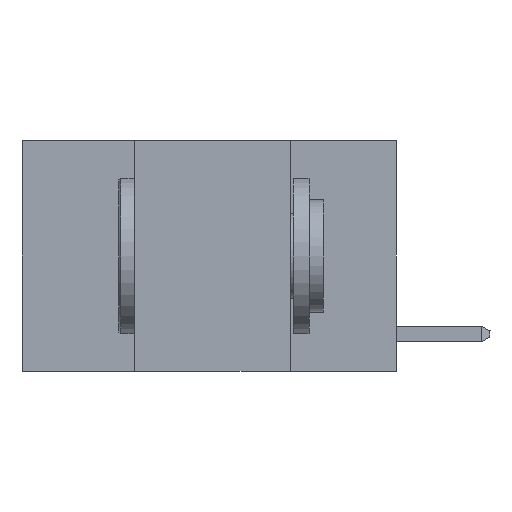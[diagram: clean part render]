
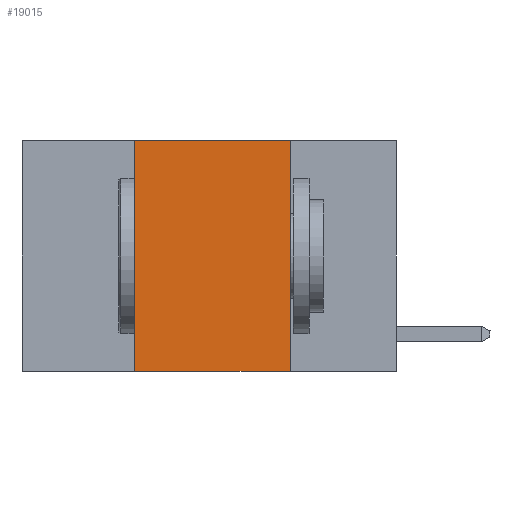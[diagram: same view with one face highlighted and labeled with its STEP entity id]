
A CAD part, left-side view. The second image highlights one B-rep face of the part: STEP entity #19015.
In plain terms, the highlighted planar face has unit normal (-1, 0, 0).
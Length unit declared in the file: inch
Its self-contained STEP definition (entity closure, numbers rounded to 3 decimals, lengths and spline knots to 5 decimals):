
#1321 = CARTESIAN_POINT ( 'NONE',  ( 0., 0.17, -0.37 ) ) ;
#1648 = EDGE_CURVE ( 'NONE', #19116, #20212, #13158, .T. ) ;
#2033 = CARTESIAN_POINT ( 'NONE',  ( 0., 0.42, -0.37 ) ) ;
#2438 = CARTESIAN_POINT ( 'NONE',  ( 0., 0.17, 0. ) ) ;
#2648 = VERTEX_POINT ( 'NONE', #1321 ) ;
#3921 = ORIENTED_EDGE ( 'NONE', *, *, #10021, .F. ) ;
#4187 = VERTEX_POINT ( 'NONE', #17325 ) ;
#4272 = ORIENTED_EDGE ( 'NONE', *, *, #1648, .F. ) ;
#4776 = VECTOR ( 'NONE', #13608, 39.37008 ) ;
#5179 = CARTESIAN_POINT ( 'NONE',  ( 0., 0.42, 0. ) ) ;
#5479 = DIRECTION ( 'NONE',  ( 0., 0., -1. ) ) ;
#6672 = PLANE ( 'NONE',  #11366 ) ;
#7063 = CARTESIAN_POINT ( 'NONE',  ( 0., 0.6, -0.37 ) ) ;
#7720 = ORIENTED_EDGE ( 'NONE', *, *, #16470, .T. ) ;
#8907 = DIRECTION ( 'NONE',  ( 0., 0., 1. ) ) ;
#8948 = CARTESIAN_POINT ( 'NONE',  ( 0., 0.42, 0. ) ) ;
#9158 = LINE ( 'NONE', #18263, #4776 ) ;
#9499 = FACE_OUTER_BOUND ( 'NONE', #11011, .T. ) ;
#10021 = EDGE_CURVE ( 'NONE', #20212, #4187, #9158, .T. ) ;
#10185 = DIRECTION ( 'NONE',  ( 1., 0., 0. ) ) ;
#10429 = VECTOR ( 'NONE', #8907, 39.37008 ) ;
#10870 = VECTOR ( 'NONE', #13972, 39.37008 ) ;
#11011 = EDGE_LOOP ( 'NONE', ( #17731, #3921, #4272, #7720 ) ) ;
#11366 = AXIS2_PLACEMENT_3D ( 'NONE', #14875, #10185, #11737 ) ;
#11737 = DIRECTION ( 'NONE',  ( 0., 0., -1. ) ) ;
#11877 = LINE ( 'NONE', #7063, #10870 ) ;
#13158 = LINE ( 'NONE', #8948, #10429 ) ;
#13287 = VECTOR ( 'NONE', #5479, 39.37008 ) ;
#13608 = DIRECTION ( 'NONE',  ( 0., -1., 0. ) ) ;
#13972 = DIRECTION ( 'NONE',  ( 0., -1., 0. ) ) ;
#14875 = CARTESIAN_POINT ( 'NONE',  ( 0., 0.6, 0. ) ) ;
#16470 = EDGE_CURVE ( 'NONE', #19116, #2648, #11877, .T. ) ;
#17325 = CARTESIAN_POINT ( 'NONE',  ( 0., 0.17, 0. ) ) ;
#17731 = ORIENTED_EDGE ( 'NONE', *, *, #18730, .F. ) ;
#18263 = CARTESIAN_POINT ( 'NONE',  ( 0., 0.6, 0. ) ) ;
#18730 = EDGE_CURVE ( 'NONE', #4187, #2648, #19944, .T. ) ;
#19015 = ADVANCED_FACE ( 'NONE', ( #9499 ), #6672, .F. ) ;
#19116 = VERTEX_POINT ( 'NONE', #2033 ) ;
#19944 = LINE ( 'NONE', #2438, #13287 ) ;
#20212 = VERTEX_POINT ( 'NONE', #5179 ) ;
